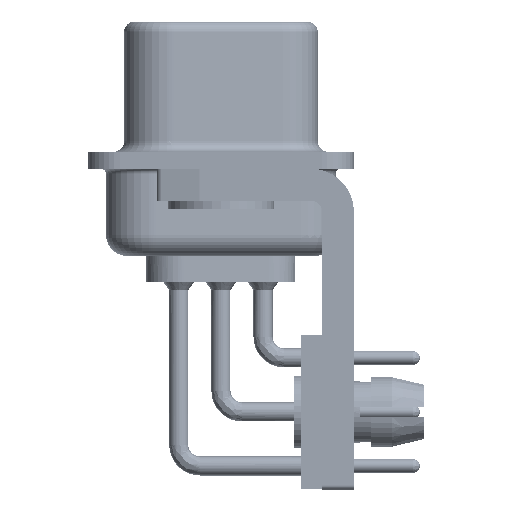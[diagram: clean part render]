
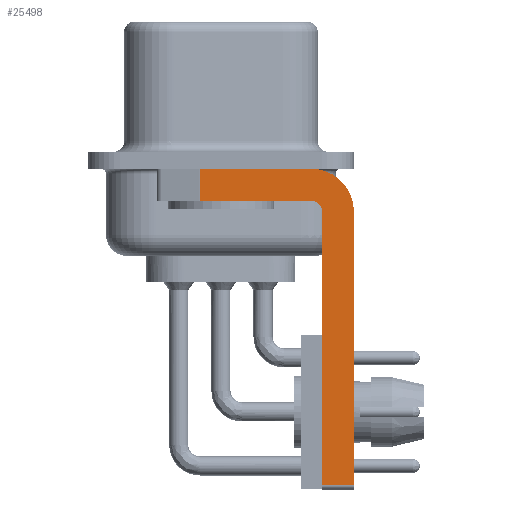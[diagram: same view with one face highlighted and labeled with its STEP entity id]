
A CAD part, left-side view. The second image highlights one B-rep face of the part: STEP entity #25498.
In plain terms, the highlighted planar face has unit normal (-1, 0, 0).
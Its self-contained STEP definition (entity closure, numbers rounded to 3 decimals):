
#1358 = DIRECTION ( 'NONE',  ( 0., 1., 0. ) ) ;
#1444 = VECTOR ( 'NONE', #32339, 1000. ) ;
#2774 = AXIS2_PLACEMENT_3D ( 'NONE', #14800, #40650, #18555 ) ;
#3019 = ORIENTED_EDGE ( 'NONE', *, *, #24935, .F. ) ;
#3182 = LINE ( 'NONE', #26786, #31422 ) ;
#3220 = CARTESIAN_POINT ( 'NONE',  ( -2.9, -4.25, -1.9 ) ) ;
#3552 = PLANE ( 'NONE',  #25821 ) ;
#3795 = FACE_OUTER_BOUND ( 'NONE', #21928, .T. ) ;
#4021 = EDGE_CURVE ( 'NONE', #44513, #41569, #3182, .T. ) ;
#4796 = CIRCLE ( 'NONE', #13447, 2. ) ;
#5429 = CARTESIAN_POINT ( 'NONE',  ( -2.9, -4.25, -0.4 ) ) ;
#5623 = EDGE_CURVE ( 'NONE', #24326, #12216, #46831, .T. ) ;
#6128 = LINE ( 'NONE', #39754, #24627 ) ;
#6913 = LINE ( 'NONE', #13468, #8074 ) ;
#7063 = CARTESIAN_POINT ( 'NONE',  ( -2.9, -4.25, -2.4 ) ) ;
#7230 = DIRECTION ( 'NONE',  ( 0., 0., -1. ) ) ;
#8074 = VECTOR ( 'NONE', #35601, 1000. ) ;
#8189 = VECTOR ( 'NONE', #9896, 1000. ) ;
#8439 = CARTESIAN_POINT ( 'NONE',  ( -2.9, 0.978, -1.9 ) ) ;
#8884 = ORIENTED_EDGE ( 'NONE', *, *, #42827, .T. ) ;
#9896 = DIRECTION ( 'NONE',  ( 0., 0., -1. ) ) ;
#10252 = CARTESIAN_POINT ( 'NONE',  ( -2.9, -4.75, -15.5 ) ) ;
#10407 = VERTEX_POINT ( 'NONE', #17448 ) ;
#10625 = EDGE_CURVE ( 'NONE', #29456, #10407, #4796, .T. ) ;
#11466 = CARTESIAN_POINT ( 'NONE',  ( -2.9, -4.25, -2.4 ) ) ;
#12216 = VERTEX_POINT ( 'NONE', #8439 ) ;
#12663 = EDGE_CURVE ( 'NONE', #46814, #24326, #15003, .T. ) ;
#13447 = AXIS2_PLACEMENT_3D ( 'NONE', #11466, #37287, #15129 ) ;
#13468 = CARTESIAN_POINT ( 'NONE',  ( -2.9, -6.25, -2.4 ) ) ;
#14800 = CARTESIAN_POINT ( 'NONE',  ( -2.9, -4.25, -2.4 ) ) ;
#15003 = CIRCLE ( 'NONE', #2774, 0.5 ) ;
#15129 = DIRECTION ( 'NONE',  ( 0., 0., -1. ) ) ;
#15225 = ORIENTED_EDGE ( 'NONE', *, *, #12663, .F. ) ;
#17063 = ORIENTED_EDGE ( 'NONE', *, *, #28950, .F. ) ;
#17325 = DIRECTION ( 'NONE',  ( 0., -1., 0. ) ) ;
#17402 = VECTOR ( 'NONE', #1358, 1000. ) ;
#17448 = CARTESIAN_POINT ( 'NONE',  ( -2.9, -6.25, -2.4 ) ) ;
#18518 = ORIENTED_EDGE ( 'NONE', *, *, #4021, .T. ) ;
#18555 = DIRECTION ( 'NONE',  ( 0., 0., 1. ) ) ;
#21928 = EDGE_LOOP ( 'NONE', ( #3019, #8884, #30430, #15225, #34416, #18518, #17063, #41259 ) ) ;
#24326 = VERTEX_POINT ( 'NONE', #3220 ) ;
#24627 = VECTOR ( 'NONE', #17325, 1000. ) ;
#24935 = EDGE_CURVE ( 'NONE', #36930, #29456, #6128, .T. ) ;
#25498 = ADVANCED_FACE ( 'NONE', ( #3795 ), #3552, .F. ) ;
#25821 = AXIS2_PLACEMENT_3D ( 'NONE', #7063, #29345, #7230 ) ;
#25989 = EDGE_CURVE ( 'NONE', #44513, #46814, #41811, .T. ) ;
#26786 = CARTESIAN_POINT ( 'NONE',  ( -2.9, -4.25, -15.25 ) ) ;
#27129 = CARTESIAN_POINT ( 'NONE',  ( -2.9, -4.25, -1.9 ) ) ;
#28950 = EDGE_CURVE ( 'NONE', #10407, #41569, #6913, .T. ) ;
#28989 = LINE ( 'NONE', #39416, #8189 ) ;
#29345 = DIRECTION ( 'NONE',  ( 1., 0., 0. ) ) ;
#29456 = VERTEX_POINT ( 'NONE', #5429 ) ;
#30430 = ORIENTED_EDGE ( 'NONE', *, *, #5623, .F. ) ;
#31422 = VECTOR ( 'NONE', #38239, 1000. ) ;
#31871 = CARTESIAN_POINT ( 'NONE',  ( -2.9, -6.25, -15.25 ) ) ;
#32339 = DIRECTION ( 'NONE',  ( 0., 0., 1. ) ) ;
#32690 = CARTESIAN_POINT ( 'NONE',  ( -2.9, 0.978, -0.4 ) ) ;
#34416 = ORIENTED_EDGE ( 'NONE', *, *, #25989, .F. ) ;
#35601 = DIRECTION ( 'NONE',  ( 0., 0., -1. ) ) ;
#36930 = VERTEX_POINT ( 'NONE', #32690 ) ;
#37287 = DIRECTION ( 'NONE',  ( 1., 0., 0. ) ) ;
#37625 = CARTESIAN_POINT ( 'NONE',  ( -2.9, -4.75, -15.25 ) ) ;
#38239 = DIRECTION ( 'NONE',  ( 0., -1., 0. ) ) ;
#39416 = CARTESIAN_POINT ( 'NONE',  ( -2.9, 0.978, -1.9 ) ) ;
#39754 = CARTESIAN_POINT ( 'NONE',  ( -2.9, 3., -0.4 ) ) ;
#40650 = DIRECTION ( 'NONE',  ( -1., 0., 0. ) ) ;
#41259 = ORIENTED_EDGE ( 'NONE', *, *, #10625, .F. ) ;
#41569 = VERTEX_POINT ( 'NONE', #31871 ) ;
#41811 = LINE ( 'NONE', #10252, #1444 ) ;
#42827 = EDGE_CURVE ( 'NONE', #36930, #12216, #28989, .T. ) ;
#44483 = CARTESIAN_POINT ( 'NONE',  ( -2.9, -4.75, -2.4 ) ) ;
#44513 = VERTEX_POINT ( 'NONE', #37625 ) ;
#46814 = VERTEX_POINT ( 'NONE', #44483 ) ;
#46831 = LINE ( 'NONE', #27129, #17402 ) ;
